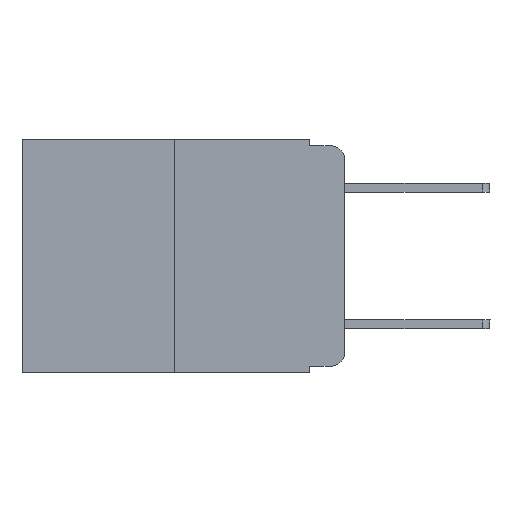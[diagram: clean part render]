
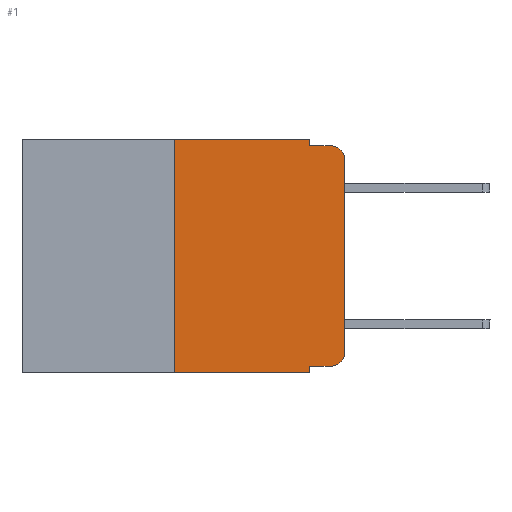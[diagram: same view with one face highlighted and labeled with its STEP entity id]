
A CAD part, left-side view. The second image highlights one B-rep face of the part: STEP entity #1.
In plain terms, the highlighted planar face has unit normal (-1, 0, 0).
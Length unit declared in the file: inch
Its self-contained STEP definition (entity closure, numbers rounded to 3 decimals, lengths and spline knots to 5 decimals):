
#1 = ADVANCED_FACE ( 'NONE', ( #135 ), #4443, .F. ) ;
#135 = FACE_OUTER_BOUND ( 'NONE', #10342, .T. ) ;
#688 = DIRECTION ( 'NONE',  ( 0., -1., 0. ) ) ;
#812 = LINE ( 'NONE', #4034, #994 ) ;
#830 = CARTESIAN_POINT ( 'NONE',  ( 0., 0.02, -0.03 ) ) ;
#864 = VERTEX_POINT ( 'NONE', #5687 ) ;
#900 = DIRECTION ( 'NONE',  ( 0., 0., 1. ) ) ;
#994 = VECTOR ( 'NONE', #9396, 39.37008 ) ;
#1179 = CARTESIAN_POINT ( 'NONE',  ( 0., 0.051, -0.333 ) ) ;
#1199 = ORIENTED_EDGE ( 'NONE', *, *, #12948, .F. ) ;
#1200 = CARTESIAN_POINT ( 'NONE',  ( 0., 0.051, -0.01 ) ) ;
#1304 = CARTESIAN_POINT ( 'NONE',  ( 0., 0.473, 0. ) ) ;
#1968 = LINE ( 'NONE', #13877, #13732 ) ;
#2028 = LINE ( 'NONE', #2999, #5075 ) ;
#2069 = LINE ( 'NONE', #13718, #6209 ) ;
#2289 = VERTEX_POINT ( 'NONE', #1179 ) ;
#2417 = CARTESIAN_POINT ( 'NONE',  ( 0., 0.25, 0. ) ) ;
#2561 = EDGE_CURVE ( 'NONE', #864, #7470, #8390, .T. ) ;
#2723 = ORIENTED_EDGE ( 'NONE', *, *, #2561, .T. ) ;
#2999 = CARTESIAN_POINT ( 'NONE',  ( 0., 0.051, 0. ) ) ;
#3090 = CARTESIAN_POINT ( 'NONE',  ( 0., 0.02, -0.01 ) ) ;
#3223 = CARTESIAN_POINT ( 'NONE',  ( 0., 0.02, -0.333 ) ) ;
#3252 = CARTESIAN_POINT ( 'NONE',  ( 0., 0.051, 0. ) ) ;
#3723 = DIRECTION ( 'NONE',  ( 0., 0., -1. ) ) ;
#3780 = DIRECTION ( 'NONE',  ( 0., 0., -1. ) ) ;
#4034 = CARTESIAN_POINT ( 'NONE',  ( 0., 0.051, -0.01 ) ) ;
#4411 = LINE ( 'NONE', #1304, #5959 ) ;
#4443 = PLANE ( 'NONE',  #11792 ) ;
#4733 = EDGE_CURVE ( 'NONE', #2289, #13453, #13672, .T. ) ;
#5075 = VECTOR ( 'NONE', #7281, 39.37008 ) ;
#5113 = DIRECTION ( 'NONE',  ( -1., 0., 0. ) ) ;
#5223 = VERTEX_POINT ( 'NONE', #3223 ) ;
#5465 = CARTESIAN_POINT ( 'NONE',  ( 0., 0., -0.03 ) ) ;
#5617 = DIRECTION ( 'NONE',  ( 0., -1., 0. ) ) ;
#5687 = CARTESIAN_POINT ( 'NONE',  ( 0., 0., -0.313 ) ) ;
#5846 = ORIENTED_EDGE ( 'NONE', *, *, #4733, .F. ) ;
#5851 = CARTESIAN_POINT ( 'NONE',  ( 0., 0.051, 0. ) ) ;
#5959 = VECTOR ( 'NONE', #5617, 39.37008 ) ;
#5962 = EDGE_CURVE ( 'NONE', #2289, #5223, #12450, .T. ) ;
#6127 = DIRECTION ( 'NONE',  ( 0., -1., 0. ) ) ;
#6209 = VECTOR ( 'NONE', #6240, 39.37008 ) ;
#6240 = DIRECTION ( 'NONE',  ( 0., 0., 1. ) ) ;
#6250 = ORIENTED_EDGE ( 'NONE', *, *, #6563, .F. ) ;
#6563 = EDGE_CURVE ( 'NONE', #12044, #8017, #2069, .T. ) ;
#7281 = DIRECTION ( 'NONE',  ( 0., 0., -1. ) ) ;
#7315 = CARTESIAN_POINT ( 'NONE',  ( 0., 0.25, -0.343 ) ) ;
#7317 = EDGE_CURVE ( 'NONE', #7470, #12477, #11742, .T. ) ;
#7470 = VERTEX_POINT ( 'NONE', #5465 ) ;
#7495 = ORIENTED_EDGE ( 'NONE', *, *, #12916, .T. ) ;
#7603 = ORIENTED_EDGE ( 'NONE', *, *, #7317, .T. ) ;
#7753 = EDGE_CURVE ( 'NONE', #8380, #12477, #812, .T. ) ;
#7888 = VECTOR ( 'NONE', #3780, 39.37008 ) ;
#7904 = VECTOR ( 'NONE', #900, 39.37008 ) ;
#7991 = VERTEX_POINT ( 'NONE', #3252 ) ;
#8017 = VERTEX_POINT ( 'NONE', #2417 ) ;
#8273 = CARTESIAN_POINT ( 'NONE',  ( 0., 0.02, -0.313 ) ) ;
#8380 = VERTEX_POINT ( 'NONE', #1200 ) ;
#8390 = LINE ( 'NONE', #10626, #7904 ) ;
#8780 = AXIS2_PLACEMENT_3D ( 'NONE', #830, #5113, #10841 ) ;
#9396 = DIRECTION ( 'NONE',  ( 0., -1., 0. ) ) ;
#10049 = EDGE_CURVE ( 'NONE', #8017, #7991, #4411, .T. ) ;
#10342 = EDGE_LOOP ( 'NONE', ( #2723, #7603, #13966, #1199, #12314, #6250, #12302, #5846, #11202, #7495 ) ) ;
#10626 = CARTESIAN_POINT ( 'NONE',  ( 0., 0., 0. ) ) ;
#10841 = DIRECTION ( 'NONE',  ( 0., 0., -1. ) ) ;
#11017 = DIRECTION ( 'NONE',  ( 1., 0., 0. ) ) ;
#11202 = ORIENTED_EDGE ( 'NONE', *, *, #5962, .T. ) ;
#11230 = CIRCLE ( 'NONE', #12141, 0.02 ) ;
#11742 = CIRCLE ( 'NONE', #8780, 0.02 ) ;
#11760 = DIRECTION ( 'NONE',  ( 0., 0., -1. ) ) ;
#11792 = AXIS2_PLACEMENT_3D ( 'NONE', #12061, #11017, #3723 ) ;
#12044 = VERTEX_POINT ( 'NONE', #7315 ) ;
#12061 = CARTESIAN_POINT ( 'NONE',  ( 0., 0.473, 0. ) ) ;
#12141 = AXIS2_PLACEMENT_3D ( 'NONE', #8273, #12608, #11760 ) ;
#12259 = CARTESIAN_POINT ( 'NONE',  ( 0., 0.051, -0.343 ) ) ;
#12302 = ORIENTED_EDGE ( 'NONE', *, *, #13634, .T. ) ;
#12314 = ORIENTED_EDGE ( 'NONE', *, *, #10049, .F. ) ;
#12450 = LINE ( 'NONE', #13524, #13436 ) ;
#12477 = VERTEX_POINT ( 'NONE', #3090 ) ;
#12608 = DIRECTION ( 'NONE',  ( -1., 0., 0. ) ) ;
#12916 = EDGE_CURVE ( 'NONE', #5223, #864, #11230, .T. ) ;
#12948 = EDGE_CURVE ( 'NONE', #7991, #8380, #2028, .T. ) ;
#13436 = VECTOR ( 'NONE', #688, 39.37008 ) ;
#13453 = VERTEX_POINT ( 'NONE', #12259 ) ;
#13524 = CARTESIAN_POINT ( 'NONE',  ( 0., 0.051, -0.333 ) ) ;
#13634 = EDGE_CURVE ( 'NONE', #12044, #13453, #1968, .T. ) ;
#13672 = LINE ( 'NONE', #5851, #7888 ) ;
#13718 = CARTESIAN_POINT ( 'NONE',  ( 0., 0.25, 0. ) ) ;
#13732 = VECTOR ( 'NONE', #6127, 39.37008 ) ;
#13877 = CARTESIAN_POINT ( 'NONE',  ( 0., 0.473, -0.343 ) ) ;
#13966 = ORIENTED_EDGE ( 'NONE', *, *, #7753, .F. ) ;
